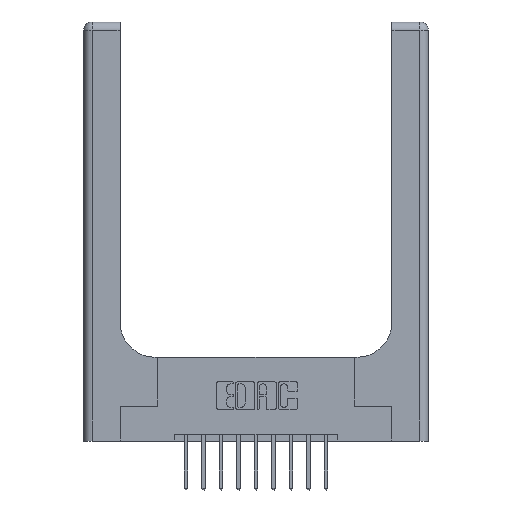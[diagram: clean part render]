
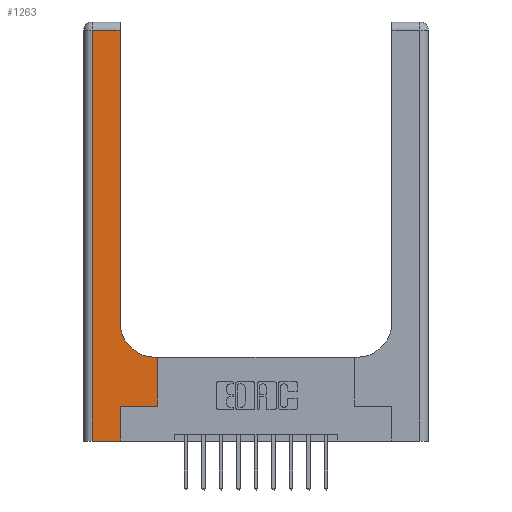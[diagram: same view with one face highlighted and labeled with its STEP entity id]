
A CAD part, top view. The second image highlights one B-rep face of the part: STEP entity #1263.
In plain terms, the highlighted planar face has unit normal (0, 0, 1).
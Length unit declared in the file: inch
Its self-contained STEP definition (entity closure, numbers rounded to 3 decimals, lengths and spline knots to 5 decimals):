
#185 = VECTOR ( 'NONE', #3866, 39.37008 ) ;
#231 = FACE_OUTER_BOUND ( 'NONE', #14347, .T. ) ;
#429 = ORIENTED_EDGE ( 'NONE', *, *, #3109, .T. ) ;
#533 = CARTESIAN_POINT ( 'NONE',  ( 0.265, 0.25, 0.37 ) ) ;
#1263 = ADVANCED_FACE ( 'NONE', ( #231 ), #4366, .F. ) ;
#1628 = AXIS2_PLACEMENT_3D ( 'NONE', #7105, #14971, #9963 ) ;
#1982 = CARTESIAN_POINT ( 'NONE',  ( 0.265, 0., 0.37 ) ) ;
#2046 = LINE ( 'NONE', #15506, #3545 ) ;
#2162 = ORIENTED_EDGE ( 'NONE', *, *, #2911, .T. ) ;
#2379 = DIRECTION ( 'NONE',  ( 0., 1., 0. ) ) ;
#2826 = LINE ( 'NONE', #4445, #3947 ) ;
#2911 = EDGE_CURVE ( 'NONE', #3901, #12526, #2826, .T. ) ;
#3109 = EDGE_CURVE ( 'NONE', #8453, #3901, #12036, .T. ) ;
#3381 = LINE ( 'NONE', #6421, #185 ) ;
#3520 = CIRCLE ( 'NONE', #1628, 0.25 ) ;
#3529 = EDGE_CURVE ( 'NONE', #7373, #6121, #2046, .T. ) ;
#3545 = VECTOR ( 'NONE', #2379, 39.37008 ) ;
#3866 = DIRECTION ( 'NONE',  ( 1., 0., 0. ) ) ;
#3882 = DIRECTION ( 'NONE',  ( -1., 0., 0. ) ) ;
#3901 = VERTEX_POINT ( 'NONE', #14497 ) ;
#3947 = VECTOR ( 'NONE', #5948, 39.37008 ) ;
#4366 = PLANE ( 'NONE',  #9164 ) ;
#4408 = ORIENTED_EDGE ( 'NONE', *, *, #12494, .T. ) ;
#4445 = CARTESIAN_POINT ( 'NONE',  ( 0., 2.94, 0.37 ) ) ;
#4685 = CARTESIAN_POINT ( 'NONE',  ( 0.06, 2.94, 0.37 ) ) ;
#4749 = EDGE_CURVE ( 'NONE', #10707, #8453, #3520, .T. ) ;
#5077 = ORIENTED_EDGE ( 'NONE', *, *, #12828, .T. ) ;
#5660 = DIRECTION ( 'NONE',  ( 0., 0., -1. ) ) ;
#5719 = CARTESIAN_POINT ( 'NONE',  ( 0.26, 0.85, 0.37 ) ) ;
#5948 = DIRECTION ( 'NONE',  ( -1., 0., 0. ) ) ;
#6121 = VERTEX_POINT ( 'NONE', #10675 ) ;
#6334 = VERTEX_POINT ( 'NONE', #12446 ) ;
#6414 = VECTOR ( 'NONE', #9444, 39.37008 ) ;
#6421 = CARTESIAN_POINT ( 'NONE',  ( 0., 0., 0.37 ) ) ;
#6682 = ORIENTED_EDGE ( 'NONE', *, *, #9338, .T. ) ;
#6948 = EDGE_CURVE ( 'NONE', #15130, #10056, #10235, .T. ) ;
#7105 = CARTESIAN_POINT ( 'NONE',  ( 0.51, 0.85, 0.37 ) ) ;
#7126 = ORIENTED_EDGE ( 'NONE', *, *, #3529, .T. ) ;
#7373 = VERTEX_POINT ( 'NONE', #14439 ) ;
#7456 = EDGE_CURVE ( 'NONE', #12526, #6334, #9245, .T. ) ;
#7678 = DIRECTION ( 'NONE',  ( 0., 1., 0. ) ) ;
#7734 = ORIENTED_EDGE ( 'NONE', *, *, #7456, .T. ) ;
#7873 = CARTESIAN_POINT ( 'NONE',  ( 0.26, 0.6, 0.37 ) ) ;
#8166 = VECTOR ( 'NONE', #14807, 39.37008 ) ;
#8433 = VECTOR ( 'NONE', #7678, 39.37008 ) ;
#8453 = VERTEX_POINT ( 'NONE', #5719 ) ;
#9164 = AXIS2_PLACEMENT_3D ( 'NONE', #10523, #5660, #3882 ) ;
#9245 = LINE ( 'NONE', #13564, #6414 ) ;
#9338 = EDGE_CURVE ( 'NONE', #6334, #15130, #3381, .T. ) ;
#9444 = DIRECTION ( 'NONE',  ( 0., -1., 0. ) ) ;
#9963 = DIRECTION ( 'NONE',  ( 1., 0., 0. ) ) ;
#10056 = VERTEX_POINT ( 'NONE', #533 ) ;
#10081 = DIRECTION ( 'NONE',  ( 0., 1., 0. ) ) ;
#10235 = LINE ( 'NONE', #12430, #12487 ) ;
#10452 = LINE ( 'NONE', #7873, #14381 ) ;
#10523 = CARTESIAN_POINT ( 'NONE',  ( 0., 3., 0.37 ) ) ;
#10675 = CARTESIAN_POINT ( 'NONE',  ( 0.528, 0.6, 0.37 ) ) ;
#10707 = VERTEX_POINT ( 'NONE', #12733 ) ;
#10824 = LINE ( 'NONE', #11106, #8166 ) ;
#11106 = CARTESIAN_POINT ( 'NONE',  ( 0.265, 0.25, 0.37 ) ) ;
#12036 = LINE ( 'NONE', #12209, #8433 ) ;
#12209 = CARTESIAN_POINT ( 'NONE',  ( 0.26, 3., 0.37 ) ) ;
#12430 = CARTESIAN_POINT ( 'NONE',  ( 0.265, 0., 0.37 ) ) ;
#12446 = CARTESIAN_POINT ( 'NONE',  ( 0.06, 0., 0.37 ) ) ;
#12487 = VECTOR ( 'NONE', #10081, 39.37008 ) ;
#12494 = EDGE_CURVE ( 'NONE', #6121, #10707, #10452, .T. ) ;
#12526 = VERTEX_POINT ( 'NONE', #4685 ) ;
#12598 = ORIENTED_EDGE ( 'NONE', *, *, #4749, .T. ) ;
#12733 = CARTESIAN_POINT ( 'NONE',  ( 0.51, 0.6, 0.37 ) ) ;
#12828 = EDGE_CURVE ( 'NONE', #10056, #7373, #10824, .T. ) ;
#13564 = CARTESIAN_POINT ( 'NONE',  ( 0.06, 3., 0.37 ) ) ;
#14347 = EDGE_LOOP ( 'NONE', ( #429, #2162, #7734, #6682, #14565, #5077, #7126, #4408, #12598 ) ) ;
#14381 = VECTOR ( 'NONE', #15324, 39.37008 ) ;
#14439 = CARTESIAN_POINT ( 'NONE',  ( 0.528, 0.25, 0.37 ) ) ;
#14497 = CARTESIAN_POINT ( 'NONE',  ( 0.26, 2.94, 0.37 ) ) ;
#14565 = ORIENTED_EDGE ( 'NONE', *, *, #6948, .T. ) ;
#14807 = DIRECTION ( 'NONE',  ( 1., 0., 0. ) ) ;
#14971 = DIRECTION ( 'NONE',  ( 0., 0., -1. ) ) ;
#15130 = VERTEX_POINT ( 'NONE', #1982 ) ;
#15324 = DIRECTION ( 'NONE',  ( -1., 0., 0. ) ) ;
#15506 = CARTESIAN_POINT ( 'NONE',  ( 0.528, 0.25, 0.37 ) ) ;
